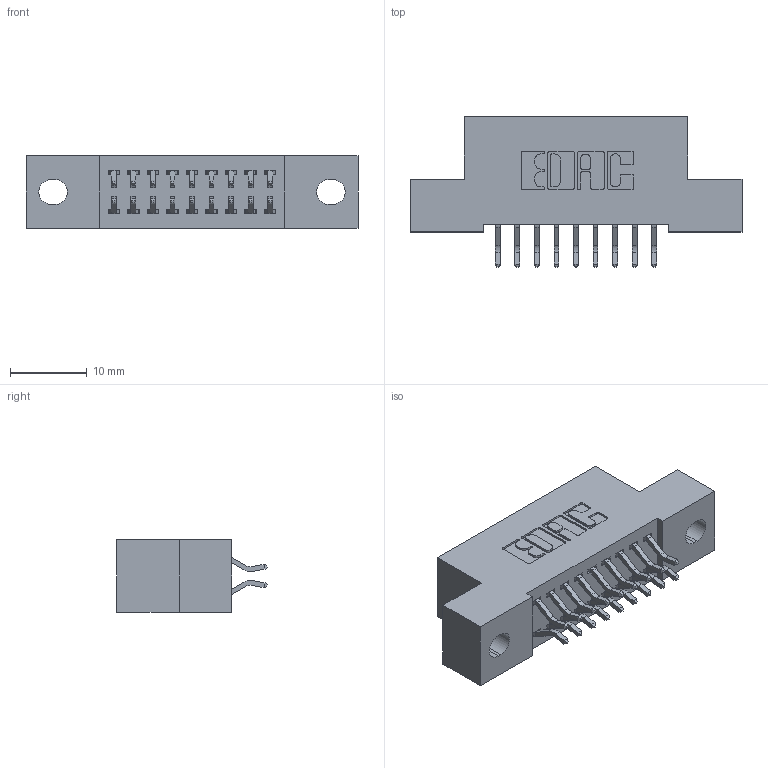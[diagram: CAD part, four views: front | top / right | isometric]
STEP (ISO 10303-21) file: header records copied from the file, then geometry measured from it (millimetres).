
FILE_DESCRIPTION (( 'STEP AP203' ), '1' );
FILE_NAME ('392-018-556-202.STEP', '2019-10-07T04:21:22', ( '' ), ( '' ), 'SwSTEP 2.0', 'SolidWorks 2016', '' );
FILE_SCHEMA (( 'CONFIG_CONTROL_DESIGN' ));
Length unit declared in the file: inch
Products named in the file (3): 342 Part_.128 Slot; 345-292-001_556 Tail; 392-018-556-202
Assembly tree (19 placements, depth 2):
  392-018-556-202
    342 Part_.128 Slot
    345-292-001_556 Tail  x18
Bounding box: 43.18 x 19.58 x 9.4 mm (x, y, z)
Volume: 3670.9 mm3; surface area: 4904.2 mm2
Topology: 19 solids, 19 shells, 1158 faces, 3425 edges, 2258 vertices
Faces by surface type: plane 790, cylinder 368
Entity records: 10281 total; most frequent: CARTESIAN_POINT 1758, ORIENTED_EDGE 1682, DIRECTION 1549, EDGE_CURVE 841, LINE 705, VECTOR 705, VERTEX_POINT 558, AXIS2_PLACEMENT_3D 422
